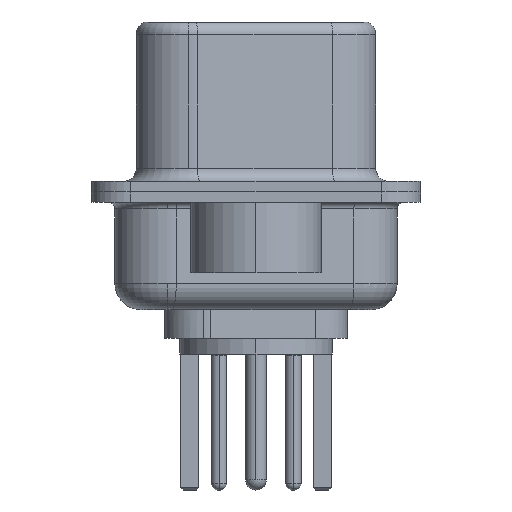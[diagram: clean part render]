
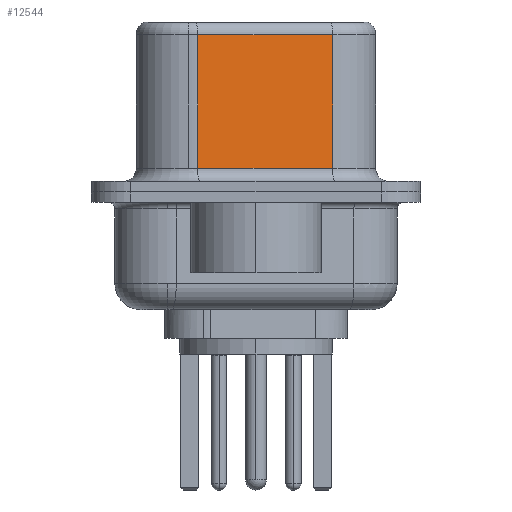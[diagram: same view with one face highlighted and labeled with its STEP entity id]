
A CAD part, left-side view. The second image highlights one B-rep face of the part: STEP entity #12544.
In plain terms, the highlighted planar face has unit normal (-0.985, -0.174, 0).
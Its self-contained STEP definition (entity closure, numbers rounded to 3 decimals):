
#241 = PLANE ( 'NONE',  #8151 ) ;
#401 = EDGE_CURVE ( 'NONE', #1700, #6406, #4916, .T. ) ;
#1278 = LINE ( 'NONE', #13996, #1760 ) ;
#1700 = VERTEX_POINT ( 'NONE', #4078 ) ;
#1760 = VECTOR ( 'NONE', #15507, 1000. ) ;
#1876 = EDGE_LOOP ( 'NONE', ( #18491, #12406, #15539, #17765 ) ) ;
#2249 = DIRECTION ( 'NONE',  ( 0., 0., -1. ) ) ;
#4078 = CARTESIAN_POINT ( 'NONE',  ( 3.655, 2.233, 6.02 ) ) ;
#4246 = EDGE_CURVE ( 'NONE', #15290, #1700, #1278, .T. ) ;
#4357 = CARTESIAN_POINT ( 'NONE',  ( 3.655, 2.233, 6.52 ) ) ;
#4916 = LINE ( 'NONE', #4357, #17880 ) ;
#6406 = VERTEX_POINT ( 'NONE', #18980 ) ;
#6635 = CARTESIAN_POINT ( 'NONE',  ( 4.565, -2.927, 6.52 ) ) ;
#6700 = DIRECTION ( 'NONE',  ( -0.174, 0.985, 0. ) ) ;
#6760 = VECTOR ( 'NONE', #16988, 1000. ) ;
#7506 = EDGE_CURVE ( 'NONE', #6406, #19674, #11011, .T. ) ;
#8151 = AXIS2_PLACEMENT_3D ( 'NONE', #6635, #16383, #6700 ) ;
#9493 = CARTESIAN_POINT ( 'NONE',  ( 4.565, -2.927, 6.02 ) ) ;
#10962 = DIRECTION ( 'NONE',  ( 0., 0., -1. ) ) ;
#11011 = LINE ( 'NONE', #17993, #6760 ) ;
#11982 = CARTESIAN_POINT ( 'NONE',  ( 4.565, -2.927, 0.9 ) ) ;
#12291 = EDGE_CURVE ( 'NONE', #15290, #19674, #20465, .T. ) ;
#12406 = ORIENTED_EDGE ( 'NONE', *, *, #4246, .T. ) ;
#12544 = ADVANCED_FACE ( 'NONE', ( #13860 ), #241, .F. ) ;
#13860 = FACE_OUTER_BOUND ( 'NONE', #1876, .T. ) ;
#13996 = CARTESIAN_POINT ( 'NONE',  ( 4.565, -2.927, 6.02 ) ) ;
#15290 = VERTEX_POINT ( 'NONE', #9493 ) ;
#15507 = DIRECTION ( 'NONE',  ( -0.174, 0.985, 0. ) ) ;
#15539 = ORIENTED_EDGE ( 'NONE', *, *, #401, .T. ) ;
#16111 = VECTOR ( 'NONE', #10962, 1000. ) ;
#16383 = DIRECTION ( 'NONE',  ( 0.985, 0.174, 0. ) ) ;
#16988 = DIRECTION ( 'NONE',  ( 0.174, -0.985, 0. ) ) ;
#17452 = CARTESIAN_POINT ( 'NONE',  ( 4.565, -2.927, 6.52 ) ) ;
#17765 = ORIENTED_EDGE ( 'NONE', *, *, #7506, .T. ) ;
#17880 = VECTOR ( 'NONE', #2249, 1000. ) ;
#17993 = CARTESIAN_POINT ( 'NONE',  ( 4.565, -2.927, 0.9 ) ) ;
#18491 = ORIENTED_EDGE ( 'NONE', *, *, #12291, .F. ) ;
#18980 = CARTESIAN_POINT ( 'NONE',  ( 3.655, 2.233, 0.9 ) ) ;
#19674 = VERTEX_POINT ( 'NONE', #11982 ) ;
#20465 = LINE ( 'NONE', #17452, #16111 ) ;
